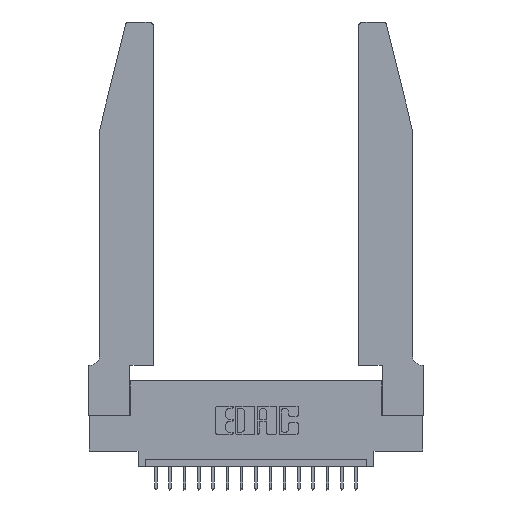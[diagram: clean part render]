
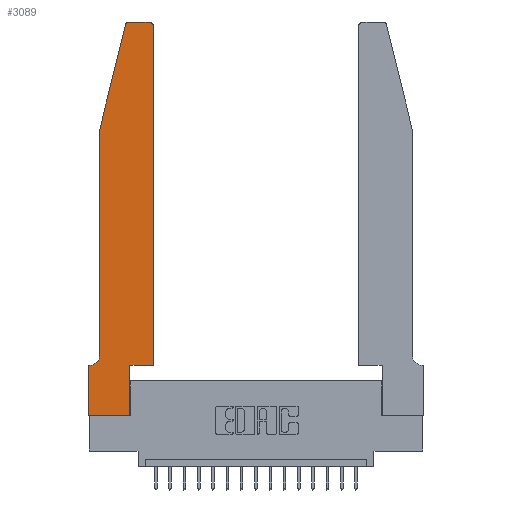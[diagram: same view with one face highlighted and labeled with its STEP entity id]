
A CAD part, top view. The second image highlights one B-rep face of the part: STEP entity #3089.
In plain terms, the highlighted planar face has unit normal (0, 0, 1).
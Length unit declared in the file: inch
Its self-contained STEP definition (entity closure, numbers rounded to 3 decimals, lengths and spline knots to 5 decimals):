
#71 = DIRECTION ( 'NONE',  ( 1., 0., 0. ) ) ;
#234 = CARTESIAN_POINT ( 'NONE',  ( 0.25487, 2.72718, 0.37 ) ) ;
#263 = PLANE ( 'NONE',  #15097 ) ;
#283 = EDGE_CURVE ( 'NONE', #16534, #18033, #12152, .T. ) ;
#542 = EDGE_CURVE ( 'NONE', #585, #3970, #19812, .T. ) ;
#585 = VERTEX_POINT ( 'NONE', #17135 ) ;
#687 = DIRECTION ( 'NONE',  ( 0., 1., 0. ) ) ;
#1133 = ORIENTED_EDGE ( 'NONE', *, *, #16942, .T. ) ;
#1223 = ORIENTED_EDGE ( 'NONE', *, *, #9184, .T. ) ;
#1772 = EDGE_CURVE ( 'NONE', #3970, #5581, #16074, .T. ) ;
#2017 = AXIS2_PLACEMENT_3D ( 'NONE', #6715, #11138, #9731 ) ;
#2048 = ORIENTED_EDGE ( 'NONE', *, *, #3556, .T. ) ;
#2056 = ORIENTED_EDGE ( 'NONE', *, *, #13567, .T. ) ;
#2124 = FACE_OUTER_BOUND ( 'NONE', #15335, .T. ) ;
#2180 = AXIS2_PLACEMENT_3D ( 'NONE', #12417, #4435, #15435 ) ;
#3089 = ADVANCED_FACE ( 'NONE', ( #2124 ), #263, .T. ) ;
#3309 = DIRECTION ( 'NONE',  ( -0.239, -0.971, 0. ) ) ;
#3358 = CARTESIAN_POINT ( 'NONE',  ( 0.0755, 0.35, 0.37 ) ) ;
#3420 = VERTEX_POINT ( 'NONE', #14396 ) ;
#3556 = EDGE_CURVE ( 'NONE', #18033, #18361, #6181, .T. ) ;
#3578 = LINE ( 'NONE', #12521, #8135 ) ;
#3714 = CARTESIAN_POINT ( 'NONE',  ( 0.284, 2.75, 0.37 ) ) ;
#3840 = CIRCLE ( 'NONE', #13018, 0.07 ) ;
#3970 = VERTEX_POINT ( 'NONE', #4925 ) ;
#4435 = DIRECTION ( 'NONE',  ( 0., 0., 1. ) ) ;
#4497 = EDGE_CURVE ( 'NONE', #3420, #10482, #13833, .T. ) ;
#4499 = VECTOR ( 'NONE', #17742, 39.37008 ) ;
#4790 = DIRECTION ( 'NONE',  ( -1., 0., 0. ) ) ;
#4925 = CARTESIAN_POINT ( 'NONE',  ( 0.4505, 2.72, 0.37 ) ) ;
#5006 = LINE ( 'NONE', #13841, #18421 ) ;
#5191 = ORIENTED_EDGE ( 'NONE', *, *, #12906, .T. ) ;
#5239 = VECTOR ( 'NONE', #687, 39.37008 ) ;
#5340 = VERTEX_POINT ( 'NONE', #3714 ) ;
#5581 = VERTEX_POINT ( 'NONE', #15310 ) ;
#6181 = LINE ( 'NONE', #8576, #5239 ) ;
#6715 = CARTESIAN_POINT ( 'NONE',  ( 0.284, 2.72, 0.37 ) ) ;
#7623 = VECTOR ( 'NONE', #15733, 39.37008 ) ;
#7916 = VERTEX_POINT ( 'NONE', #10595 ) ;
#8059 = VECTOR ( 'NONE', #11917, 39.37008 ) ;
#8135 = VECTOR ( 'NONE', #3309, 39.37008 ) ;
#8143 = DIRECTION ( 'NONE',  ( -1., 0., 0. ) ) ;
#8151 = CARTESIAN_POINT ( 'NONE',  ( 0.2865, 0.35, 0.37 ) ) ;
#8576 = CARTESIAN_POINT ( 'NONE',  ( 0.2865, 0.35, 0.37 ) ) ;
#8902 = EDGE_CURVE ( 'NONE', #7916, #19435, #10980, .T. ) ;
#8925 = EDGE_CURVE ( 'NONE', #5581, #5340, #5006, .T. ) ;
#8927 = CARTESIAN_POINT ( 'NONE',  ( 0., 0.35, 0.37 ) ) ;
#8958 = CARTESIAN_POINT ( 'NONE',  ( 0., 0., 0.37 ) ) ;
#9184 = EDGE_CURVE ( 'NONE', #18361, #585, #18158, .T. ) ;
#9731 = DIRECTION ( 'NONE',  ( 1., 0., 0. ) ) ;
#9864 = LINE ( 'NONE', #18029, #12299 ) ;
#10482 = VERTEX_POINT ( 'NONE', #15148 ) ;
#10595 = CARTESIAN_POINT ( 'NONE',  ( 0.0055, 0.35, 0.37 ) ) ;
#10934 = CARTESIAN_POINT ( 'NONE',  ( 0., 0.35, 0.37 ) ) ;
#10980 = LINE ( 'NONE', #3358, #7623 ) ;
#11138 = DIRECTION ( 'NONE',  ( 0., 0., 1. ) ) ;
#11242 = CARTESIAN_POINT ( 'NONE',  ( 0.0055, 0.42, 0.37 ) ) ;
#11857 = VECTOR ( 'NONE', #14278, 39.37008 ) ;
#11887 = CARTESIAN_POINT ( 'NONE',  ( 0.0755, 2., 0.37 ) ) ;
#11917 = DIRECTION ( 'NONE',  ( 1., 0., 0. ) ) ;
#11953 = DIRECTION ( 'NONE',  ( 0., -1., 0. ) ) ;
#12152 = LINE ( 'NONE', #8958, #8059 ) ;
#12299 = VECTOR ( 'NONE', #16462, 39.37008 ) ;
#12417 = CARTESIAN_POINT ( 'NONE',  ( 0.4205, 2.72, 0.37 ) ) ;
#12465 = CARTESIAN_POINT ( 'NONE',  ( 0.4505, 0.35, 0.37 ) ) ;
#12521 = CARTESIAN_POINT ( 'NONE',  ( 0.0755, 2., 0.37 ) ) ;
#12906 = EDGE_CURVE ( 'NONE', #19435, #16534, #9864, .T. ) ;
#12948 = CARTESIAN_POINT ( 'NONE',  ( 0.4505, 0.35, 0.37 ) ) ;
#13018 = AXIS2_PLACEMENT_3D ( 'NONE', #11242, #15754, #8143 ) ;
#13135 = ORIENTED_EDGE ( 'NONE', *, *, #283, .T. ) ;
#13324 = ORIENTED_EDGE ( 'NONE', *, *, #1772, .T. ) ;
#13567 = EDGE_CURVE ( 'NONE', #10482, #7916, #3840, .T. ) ;
#13588 = ORIENTED_EDGE ( 'NONE', *, *, #8925, .T. ) ;
#13833 = LINE ( 'NONE', #11887, #15261 ) ;
#13841 = CARTESIAN_POINT ( 'NONE',  ( 0.2605, 2.75, 0.37 ) ) ;
#14039 = DIRECTION ( 'NONE',  ( 0., 0., 1. ) ) ;
#14278 = DIRECTION ( 'NONE',  ( 0., 1., 0. ) ) ;
#14396 = CARTESIAN_POINT ( 'NONE',  ( 0.0755, 2., 0.37 ) ) ;
#14969 = ORIENTED_EDGE ( 'NONE', *, *, #4497, .T. ) ;
#15097 = AXIS2_PLACEMENT_3D ( 'NONE', #10934, #14039, #71 ) ;
#15148 = CARTESIAN_POINT ( 'NONE',  ( 0.0755, 0.42, 0.37 ) ) ;
#15261 = VECTOR ( 'NONE', #11953, 39.37008 ) ;
#15310 = CARTESIAN_POINT ( 'NONE',  ( 0.4205, 2.75, 0.37 ) ) ;
#15335 = EDGE_LOOP ( 'NONE', ( #13588, #1133, #19815, #14969, #2056, #15412, #5191, #13135, #2048, #1223, #18627, #13324 ) ) ;
#15412 = ORIENTED_EDGE ( 'NONE', *, *, #8902, .T. ) ;
#15435 = DIRECTION ( 'NONE',  ( 1., 0., 0. ) ) ;
#15733 = DIRECTION ( 'NONE',  ( -1., 0., 0. ) ) ;
#15754 = DIRECTION ( 'NONE',  ( 0., 0., -1. ) ) ;
#16072 = CIRCLE ( 'NONE', #2017, 0.03 ) ;
#16074 = CIRCLE ( 'NONE', #2180, 0.03 ) ;
#16296 = CARTESIAN_POINT ( 'NONE',  ( 0.2865, 0., 0.37 ) ) ;
#16462 = DIRECTION ( 'NONE',  ( 0., -1., 0. ) ) ;
#16534 = VERTEX_POINT ( 'NONE', #19488 ) ;
#16942 = EDGE_CURVE ( 'NONE', #5340, #18913, #16072, .T. ) ;
#17072 = EDGE_CURVE ( 'NONE', #18913, #3420, #3578, .T. ) ;
#17135 = CARTESIAN_POINT ( 'NONE',  ( 0.4505, 0.35, 0.37 ) ) ;
#17742 = DIRECTION ( 'NONE',  ( 1., 0., 0. ) ) ;
#18029 = CARTESIAN_POINT ( 'NONE',  ( 0., 0., 0.37 ) ) ;
#18033 = VERTEX_POINT ( 'NONE', #16296 ) ;
#18158 = LINE ( 'NONE', #12948, #4499 ) ;
#18361 = VERTEX_POINT ( 'NONE', #8151 ) ;
#18421 = VECTOR ( 'NONE', #4790, 39.37008 ) ;
#18627 = ORIENTED_EDGE ( 'NONE', *, *, #542, .T. ) ;
#18913 = VERTEX_POINT ( 'NONE', #234 ) ;
#19435 = VERTEX_POINT ( 'NONE', #8927 ) ;
#19488 = CARTESIAN_POINT ( 'NONE',  ( 0., 0., 0.37 ) ) ;
#19812 = LINE ( 'NONE', #12465, #11857 ) ;
#19815 = ORIENTED_EDGE ( 'NONE', *, *, #17072, .T. ) ;
